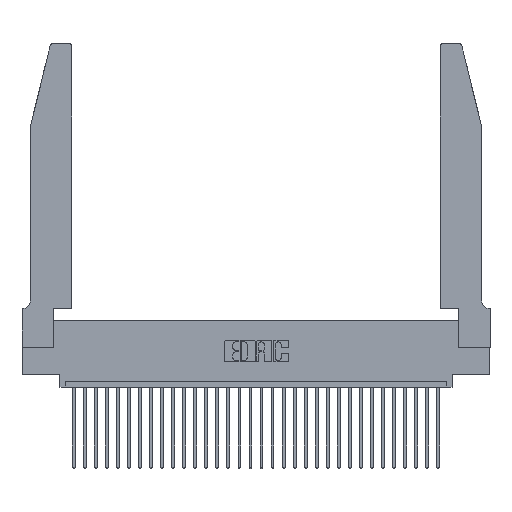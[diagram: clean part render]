
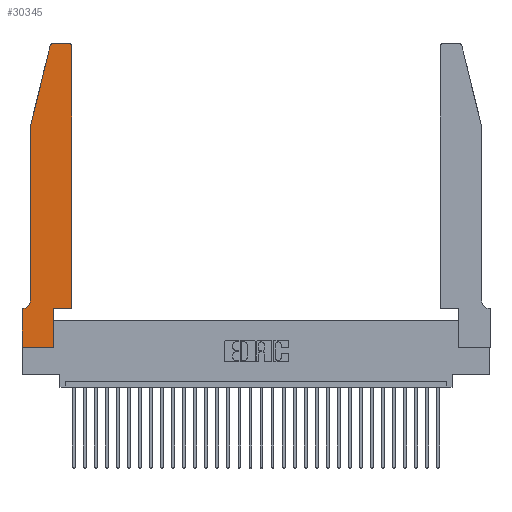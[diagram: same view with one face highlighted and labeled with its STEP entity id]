
A CAD part, top view. The second image highlights one B-rep face of the part: STEP entity #30345.
In plain terms, the highlighted planar face has unit normal (0, 0, 1).
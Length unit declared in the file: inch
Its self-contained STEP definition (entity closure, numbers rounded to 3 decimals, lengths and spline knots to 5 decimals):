
#185 = VERTEX_POINT ( 'NONE', #14735 ) ;
#557 = EDGE_CURVE ( 'NONE', #27077, #185, #27955, .T. ) ;
#727 = CARTESIAN_POINT ( 'NONE',  ( 0., 0., 0.37 ) ) ;
#935 = CARTESIAN_POINT ( 'NONE',  ( 0.284, 2.72, 0.37 ) ) ;
#986 = VERTEX_POINT ( 'NONE', #14891 ) ;
#1115 = CARTESIAN_POINT ( 'NONE',  ( 0.4505, 2.72, 0.37 ) ) ;
#1324 = CARTESIAN_POINT ( 'NONE',  ( 0., 0., 0.37 ) ) ;
#1462 = AXIS2_PLACEMENT_3D ( 'NONE', #25644, #9673, #12925 ) ;
#1627 = VECTOR ( 'NONE', #9304, 39.37008 ) ;
#1652 = CARTESIAN_POINT ( 'NONE',  ( 0., 0., 0.37 ) ) ;
#2149 = AXIS2_PLACEMENT_3D ( 'NONE', #935, #30024, #5843 ) ;
#3223 = ORIENTED_EDGE ( 'NONE', *, *, #29533, .T. ) ;
#3311 = CARTESIAN_POINT ( 'NONE',  ( 0.2865, 0.35, 0.37 ) ) ;
#3704 = VERTEX_POINT ( 'NONE', #27938 ) ;
#3735 = VERTEX_POINT ( 'NONE', #25283 ) ;
#4009 = EDGE_CURVE ( 'NONE', #7381, #16774, #21626, .T. ) ;
#4032 = CARTESIAN_POINT ( 'NONE',  ( 0.284, 2.75, 0.37 ) ) ;
#4155 = ORIENTED_EDGE ( 'NONE', *, *, #22844, .T. ) ;
#4300 = CARTESIAN_POINT ( 'NONE',  ( 0., 0.35, 0.37 ) ) ;
#4344 = EDGE_CURVE ( 'NONE', #16774, #3735, #23517, .T. ) ;
#4731 = VECTOR ( 'NONE', #9141, 39.37008 ) ;
#4835 = VECTOR ( 'NONE', #21336, 39.37008 ) ;
#5676 = CIRCLE ( 'NONE', #2149, 0.03 ) ;
#5828 = LINE ( 'NONE', #1324, #10802 ) ;
#5843 = DIRECTION ( 'NONE',  ( 1., 0., 0. ) ) ;
#6719 = ORIENTED_EDGE ( 'NONE', *, *, #20015, .T. ) ;
#6909 = ORIENTED_EDGE ( 'NONE', *, *, #10300, .T. ) ;
#7037 = LINE ( 'NONE', #26062, #4731 ) ;
#7052 = CARTESIAN_POINT ( 'NONE',  ( 0.0755, 2., 0.37 ) ) ;
#7381 = VERTEX_POINT ( 'NONE', #23566 ) ;
#7666 = ORIENTED_EDGE ( 'NONE', *, *, #557, .T. ) ;
#8485 = DIRECTION ( 'NONE',  ( 0., -1., 0. ) ) ;
#8966 = VERTEX_POINT ( 'NONE', #26600 ) ;
#9141 = DIRECTION ( 'NONE',  ( -1., 0., 0. ) ) ;
#9234 = DIRECTION ( 'NONE',  ( 1., 0., 0. ) ) ;
#9304 = DIRECTION ( 'NONE',  ( 0., 1., 0. ) ) ;
#9411 = CARTESIAN_POINT ( 'NONE',  ( 0.0755, 0.35, 0.37 ) ) ;
#9499 = EDGE_CURVE ( 'NONE', #8966, #29303, #19216, .T. ) ;
#9673 = DIRECTION ( 'NONE',  ( 0., 0., 1. ) ) ;
#10300 = EDGE_CURVE ( 'NONE', #29303, #986, #10762, .T. ) ;
#10729 = ORIENTED_EDGE ( 'NONE', *, *, #25085, .T. ) ;
#10762 = CIRCLE ( 'NONE', #1462, 0.03 ) ;
#10802 = VECTOR ( 'NONE', #8485, 39.37008 ) ;
#10920 = EDGE_CURVE ( 'NONE', #3735, #11209, #30878, .T. ) ;
#11209 = VERTEX_POINT ( 'NONE', #21007 ) ;
#12507 = ORIENTED_EDGE ( 'NONE', *, *, #26997, .T. ) ;
#12925 = DIRECTION ( 'NONE',  ( 1., 0., 0. ) ) ;
#13078 = CARTESIAN_POINT ( 'NONE',  ( 0.0755, 2., 0.37 ) ) ;
#13696 = ORIENTED_EDGE ( 'NONE', *, *, #4009, .T. ) ;
#14465 = VERTEX_POINT ( 'NONE', #3311 ) ;
#14481 = DIRECTION ( 'NONE',  ( -1., 0., 0. ) ) ;
#14735 = CARTESIAN_POINT ( 'NONE',  ( 0.2865, 0., 0.37 ) ) ;
#14793 = ORIENTED_EDGE ( 'NONE', *, *, #10920, .T. ) ;
#14891 = CARTESIAN_POINT ( 'NONE',  ( 0.4205, 2.75, 0.37 ) ) ;
#16124 = DIRECTION ( 'NONE',  ( 1., 0., 0. ) ) ;
#16770 = DIRECTION ( 'NONE',  ( -1., 0., 0. ) ) ;
#16774 = VERTEX_POINT ( 'NONE', #27888 ) ;
#17493 = AXIS2_PLACEMENT_3D ( 'NONE', #4300, #23813, #9234 ) ;
#18808 = DIRECTION ( 'NONE',  ( 0., 0., -1. ) ) ;
#19216 = LINE ( 'NONE', #26021, #1627 ) ;
#19257 = VERTEX_POINT ( 'NONE', #4032 ) ;
#19340 = VECTOR ( 'NONE', #30943, 39.37008 ) ;
#20015 = EDGE_CURVE ( 'NONE', #185, #14465, #28065, .T. ) ;
#20559 = DIRECTION ( 'NONE',  ( -0.239, -0.971, 0. ) ) ;
#21007 = CARTESIAN_POINT ( 'NONE',  ( 0.0055, 0.35, 0.37 ) ) ;
#21087 = FACE_OUTER_BOUND ( 'NONE', #22920, .T. ) ;
#21336 = DIRECTION ( 'NONE',  ( 0., -1., 0. ) ) ;
#21563 = CARTESIAN_POINT ( 'NONE',  ( 0.0055, 0.42, 0.37 ) ) ;
#21626 = LINE ( 'NONE', #13078, #22786 ) ;
#22500 = AXIS2_PLACEMENT_3D ( 'NONE', #21563, #18808, #16770 ) ;
#22786 = VECTOR ( 'NONE', #20559, 39.37008 ) ;
#22844 = EDGE_CURVE ( 'NONE', #14465, #8966, #24153, .T. ) ;
#22920 = EDGE_LOOP ( 'NONE', ( #3223, #12507, #13696, #24777, #14793, #10729, #27199, #7666, #6719, #4155, #25750, #6909 ) ) ;
#23517 = LINE ( 'NONE', #7052, #4835 ) ;
#23566 = CARTESIAN_POINT ( 'NONE',  ( 0.25487, 2.72718, 0.37 ) ) ;
#23615 = DIRECTION ( 'NONE',  ( 1., 0., 0. ) ) ;
#23813 = DIRECTION ( 'NONE',  ( 0., 0., 1. ) ) ;
#24153 = LINE ( 'NONE', #30689, #28329 ) ;
#24777 = ORIENTED_EDGE ( 'NONE', *, *, #4344, .T. ) ;
#24898 = VECTOR ( 'NONE', #23615, 39.37008 ) ;
#25085 = EDGE_CURVE ( 'NONE', #11209, #3704, #31562, .T. ) ;
#25283 = CARTESIAN_POINT ( 'NONE',  ( 0.0755, 0.42, 0.37 ) ) ;
#25644 = CARTESIAN_POINT ( 'NONE',  ( 0.4205, 2.72, 0.37 ) ) ;
#25750 = ORIENTED_EDGE ( 'NONE', *, *, #9499, .T. ) ;
#26021 = CARTESIAN_POINT ( 'NONE',  ( 0.4505, 0.35, 0.37 ) ) ;
#26062 = CARTESIAN_POINT ( 'NONE',  ( 0.2605, 2.75, 0.37 ) ) ;
#26600 = CARTESIAN_POINT ( 'NONE',  ( 0.4505, 0.35, 0.37 ) ) ;
#26997 = EDGE_CURVE ( 'NONE', #19257, #7381, #5676, .T. ) ;
#27077 = VERTEX_POINT ( 'NONE', #727 ) ;
#27199 = ORIENTED_EDGE ( 'NONE', *, *, #30091, .T. ) ;
#27888 = CARTESIAN_POINT ( 'NONE',  ( 0.0755, 2., 0.37 ) ) ;
#27938 = CARTESIAN_POINT ( 'NONE',  ( 0., 0.35, 0.37 ) ) ;
#27955 = LINE ( 'NONE', #1652, #24898 ) ;
#28065 = LINE ( 'NONE', #30839, #19340 ) ;
#28329 = VECTOR ( 'NONE', #16124, 39.37008 ) ;
#29303 = VERTEX_POINT ( 'NONE', #1115 ) ;
#29533 = EDGE_CURVE ( 'NONE', #986, #19257, #7037, .T. ) ;
#29678 = VECTOR ( 'NONE', #14481, 39.37008 ) ;
#30024 = DIRECTION ( 'NONE',  ( 0., 0., 1. ) ) ;
#30091 = EDGE_CURVE ( 'NONE', #3704, #27077, #5828, .T. ) ;
#30345 = ADVANCED_FACE ( 'NONE', ( #21087 ), #30831, .T. ) ;
#30689 = CARTESIAN_POINT ( 'NONE',  ( 0.4505, 0.35, 0.37 ) ) ;
#30831 = PLANE ( 'NONE',  #17493 ) ;
#30839 = CARTESIAN_POINT ( 'NONE',  ( 0.2865, 0.35, 0.37 ) ) ;
#30878 = CIRCLE ( 'NONE', #22500, 0.07 ) ;
#30943 = DIRECTION ( 'NONE',  ( 0., 1., 0. ) ) ;
#31562 = LINE ( 'NONE', #9411, #29678 ) ;
